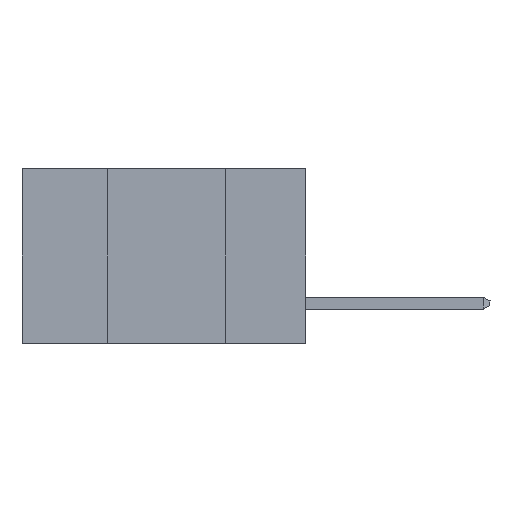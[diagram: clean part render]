
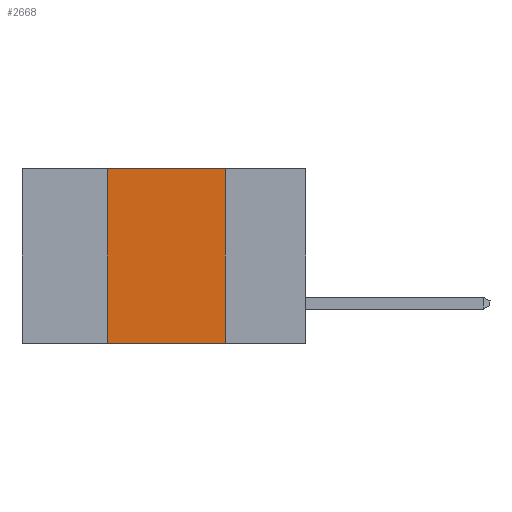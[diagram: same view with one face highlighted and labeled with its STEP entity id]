
A CAD part, left-side view. The second image highlights one B-rep face of the part: STEP entity #2668.
In plain terms, the highlighted planar face has unit normal (-1, 0, 0).
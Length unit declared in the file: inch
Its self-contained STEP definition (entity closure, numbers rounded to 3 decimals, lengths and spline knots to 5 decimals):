
#765 = LINE ( 'NONE', #14413, #17663 ) ;
#1837 = EDGE_CURVE ( 'NONE', #2777, #3828, #17385, .T. ) ;
#2015 = CARTESIAN_POINT ( 'NONE',  ( 0., 0.6, 0. ) ) ;
#2025 = ORIENTED_EDGE ( 'NONE', *, *, #10466, .F. ) ;
#2668 = ADVANCED_FACE ( 'NONE', ( #18036 ), #3098, .F. ) ;
#2673 = ORIENTED_EDGE ( 'NONE', *, *, #15205, .F. ) ;
#2777 = VERTEX_POINT ( 'NONE', #16500 ) ;
#2829 = VECTOR ( 'NONE', #16742, 39.37008 ) ;
#3098 = PLANE ( 'NONE',  #4191 ) ;
#3552 = CARTESIAN_POINT ( 'NONE',  ( 0., 0.42, 0. ) ) ;
#3591 = CARTESIAN_POINT ( 'NONE',  ( 0., 0.17, -0.37 ) ) ;
#3828 = VERTEX_POINT ( 'NONE', #3591 ) ;
#4191 = AXIS2_PLACEMENT_3D ( 'NONE', #2015, #12650, #12915 ) ;
#4934 = CARTESIAN_POINT ( 'NONE',  ( 0., 0.6, -0.37 ) ) ;
#6866 = EDGE_CURVE ( 'NONE', #9701, #3828, #7350, .T. ) ;
#7350 = LINE ( 'NONE', #13591, #2829 ) ;
#9701 = VERTEX_POINT ( 'NONE', #12615 ) ;
#9909 = CARTESIAN_POINT ( 'NONE',  ( 0., 0.42, 0. ) ) ;
#10234 = ORIENTED_EDGE ( 'NONE', *, *, #1837, .T. ) ;
#10416 = VERTEX_POINT ( 'NONE', #9909 ) ;
#10430 = VECTOR ( 'NONE', #18691, 39.37008 ) ;
#10466 = EDGE_CURVE ( 'NONE', #2777, #10416, #10700, .T. ) ;
#10700 = LINE ( 'NONE', #3552, #16647 ) ;
#12615 = CARTESIAN_POINT ( 'NONE',  ( 0., 0.17, 0. ) ) ;
#12650 = DIRECTION ( 'NONE',  ( 1., 0., 0. ) ) ;
#12706 = DIRECTION ( 'NONE',  ( 0., 0., 1. ) ) ;
#12915 = DIRECTION ( 'NONE',  ( 0., 0., -1. ) ) ;
#13591 = CARTESIAN_POINT ( 'NONE',  ( 0., 0.17, 0. ) ) ;
#14413 = CARTESIAN_POINT ( 'NONE',  ( 0., 0.6, 0. ) ) ;
#15205 = EDGE_CURVE ( 'NONE', #10416, #9701, #765, .T. ) ;
#16500 = CARTESIAN_POINT ( 'NONE',  ( 0., 0.42, -0.37 ) ) ;
#16647 = VECTOR ( 'NONE', #12706, 39.37008 ) ;
#16742 = DIRECTION ( 'NONE',  ( 0., 0., -1. ) ) ;
#17385 = LINE ( 'NONE', #4934, #10430 ) ;
#17663 = VECTOR ( 'NONE', #19017, 39.37008 ) ;
#18036 = FACE_OUTER_BOUND ( 'NONE', #19061, .T. ) ;
#18691 = DIRECTION ( 'NONE',  ( 0., -1., 0. ) ) ;
#19017 = DIRECTION ( 'NONE',  ( 0., -1., 0. ) ) ;
#19061 = EDGE_LOOP ( 'NONE', ( #19600, #2673, #2025, #10234 ) ) ;
#19600 = ORIENTED_EDGE ( 'NONE', *, *, #6866, .F. ) ;
